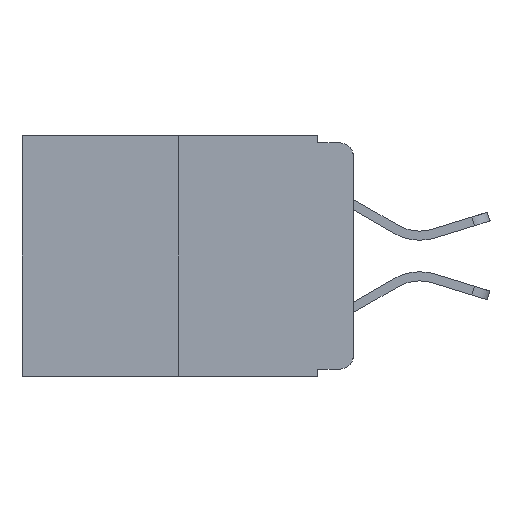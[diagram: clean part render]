
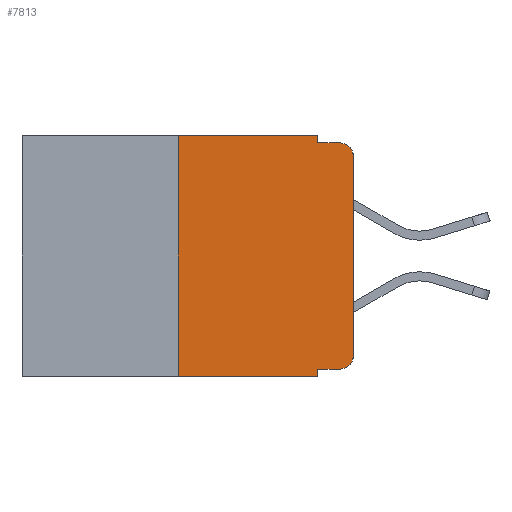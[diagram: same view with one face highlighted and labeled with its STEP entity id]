
A CAD part, left-side view. The second image highlights one B-rep face of the part: STEP entity #7813.
In plain terms, the highlighted planar face has unit normal (-1, 0, 0).
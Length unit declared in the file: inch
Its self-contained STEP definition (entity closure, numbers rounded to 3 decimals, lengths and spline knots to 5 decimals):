
#68 = AXIS2_PLACEMENT_3D ( 'NONE', #7513, #20662, #9401 ) ;
#79 = VECTOR ( 'NONE', #5910, 39.37008 ) ;
#618 = ORIENTED_EDGE ( 'NONE', *, *, #15214, .T. ) ;
#632 = DIRECTION ( 'NONE',  ( 0., -1., 0. ) ) ;
#761 = LINE ( 'NONE', #13624, #79 ) ;
#1089 = DIRECTION ( 'NONE',  ( 0., 0., -1. ) ) ;
#1434 = CIRCLE ( 'NONE', #7834, 0.02 ) ;
#1561 = EDGE_CURVE ( 'NONE', #3137, #16439, #16913, .T. ) ;
#1835 = LINE ( 'NONE', #22205, #12300 ) ;
#1865 = EDGE_CURVE ( 'NONE', #13426, #11484, #1434, .T. ) ;
#2576 = CARTESIAN_POINT ( 'NONE',  ( 0., 0.25, -0.343 ) ) ;
#2655 = CARTESIAN_POINT ( 'NONE',  ( 0., 0., 0. ) ) ;
#2921 = VECTOR ( 'NONE', #24233, 39.37008 ) ;
#3137 = VERTEX_POINT ( 'NONE', #23814 ) ;
#3278 = LINE ( 'NONE', #16063, #17871 ) ;
#3741 = ORIENTED_EDGE ( 'NONE', *, *, #1561, .T. ) ;
#3754 = AXIS2_PLACEMENT_3D ( 'NONE', #3768, #17104, #5752 ) ;
#3768 = CARTESIAN_POINT ( 'NONE',  ( 0., 0.473, 0. ) ) ;
#4059 = ORIENTED_EDGE ( 'NONE', *, *, #12887, .F. ) ;
#4904 = FACE_OUTER_BOUND ( 'NONE', #19486, .T. ) ;
#4918 = CARTESIAN_POINT ( 'NONE',  ( 0., 0.02, -0.01 ) ) ;
#5603 = ORIENTED_EDGE ( 'NONE', *, *, #19081, .T. ) ;
#5752 = DIRECTION ( 'NONE',  ( 0., 0., -1. ) ) ;
#5910 = DIRECTION ( 'NONE',  ( 0., 0., 1. ) ) ;
#6011 = VECTOR ( 'NONE', #632, 39.37008 ) ;
#6582 = DIRECTION ( 'NONE',  ( 0., 0., 1. ) ) ;
#6622 = LINE ( 'NONE', #14432, #6011 ) ;
#6765 = VERTEX_POINT ( 'NONE', #15989 ) ;
#7513 = CARTESIAN_POINT ( 'NONE',  ( 0., 0.02, -0.313 ) ) ;
#7595 = LINE ( 'NONE', #2655, #11539 ) ;
#7813 = ADVANCED_FACE ( 'NONE', ( #4904 ), #11496, .F. ) ;
#7834 = AXIS2_PLACEMENT_3D ( 'NONE', #23665, #23700, #21251 ) ;
#8142 = LINE ( 'NONE', #11283, #2921 ) ;
#9237 = VERTEX_POINT ( 'NONE', #12190 ) ;
#9401 = DIRECTION ( 'NONE',  ( 0., 0., -1. ) ) ;
#9455 = EDGE_CURVE ( 'NONE', #14515, #6765, #12429, .T. ) ;
#10920 = CARTESIAN_POINT ( 'NONE',  ( 0., 0.473, 0. ) ) ;
#11263 = CARTESIAN_POINT ( 'NONE',  ( 0., 0.02, -0.333 ) ) ;
#11283 = CARTESIAN_POINT ( 'NONE',  ( 0., 0.473, -0.343 ) ) ;
#11401 = VECTOR ( 'NONE', #16512, 39.37008 ) ;
#11484 = VERTEX_POINT ( 'NONE', #4918 ) ;
#11496 = PLANE ( 'NONE',  #3754 ) ;
#11539 = VECTOR ( 'NONE', #6582, 39.37008 ) ;
#11835 = VECTOR ( 'NONE', #12847, 39.37008 ) ;
#12190 = CARTESIAN_POINT ( 'NONE',  ( 0., 0., -0.313 ) ) ;
#12300 = VECTOR ( 'NONE', #1089, 39.37008 ) ;
#12429 = LINE ( 'NONE', #10920, #11835 ) ;
#12629 = VERTEX_POINT ( 'NONE', #14851 ) ;
#12847 = DIRECTION ( 'NONE',  ( 0., -1., 0. ) ) ;
#12887 = EDGE_CURVE ( 'NONE', #14483, #14515, #761, .T. ) ;
#13285 = CARTESIAN_POINT ( 'NONE',  ( 0., 0., -0.03 ) ) ;
#13357 = CARTESIAN_POINT ( 'NONE',  ( 0., 0.051, -0.333 ) ) ;
#13426 = VERTEX_POINT ( 'NONE', #13285 ) ;
#13624 = CARTESIAN_POINT ( 'NONE',  ( 0., 0.25, 0. ) ) ;
#13991 = EDGE_CURVE ( 'NONE', #3137, #16441, #1835, .T. ) ;
#14291 = CARTESIAN_POINT ( 'NONE',  ( 0., 0.25, 0. ) ) ;
#14432 = CARTESIAN_POINT ( 'NONE',  ( 0., 0.051, -0.01 ) ) ;
#14483 = VERTEX_POINT ( 'NONE', #2576 ) ;
#14515 = VERTEX_POINT ( 'NONE', #14291 ) ;
#14851 = CARTESIAN_POINT ( 'NONE',  ( 0., 0.051, -0.01 ) ) ;
#15214 = EDGE_CURVE ( 'NONE', #16439, #9237, #17437, .T. ) ;
#15421 = ORIENTED_EDGE ( 'NONE', *, *, #9455, .F. ) ;
#15921 = ORIENTED_EDGE ( 'NONE', *, *, #18143, .T. ) ;
#15989 = CARTESIAN_POINT ( 'NONE',  ( 0., 0.051, 0. ) ) ;
#16063 = CARTESIAN_POINT ( 'NONE',  ( 0., 0.051, 0. ) ) ;
#16439 = VERTEX_POINT ( 'NONE', #11263 ) ;
#16441 = VERTEX_POINT ( 'NONE', #18652 ) ;
#16512 = DIRECTION ( 'NONE',  ( 0., -1., 0. ) ) ;
#16588 = ORIENTED_EDGE ( 'NONE', *, *, #18829, .F. ) ;
#16913 = LINE ( 'NONE', #13357, #11401 ) ;
#17104 = DIRECTION ( 'NONE',  ( 1., 0., 0. ) ) ;
#17163 = ORIENTED_EDGE ( 'NONE', *, *, #13991, .F. ) ;
#17437 = CIRCLE ( 'NONE', #68, 0.02 ) ;
#17871 = VECTOR ( 'NONE', #21653, 39.37008 ) ;
#18143 = EDGE_CURVE ( 'NONE', #9237, #13426, #7595, .T. ) ;
#18652 = CARTESIAN_POINT ( 'NONE',  ( 0., 0.051, -0.343 ) ) ;
#18829 = EDGE_CURVE ( 'NONE', #6765, #12629, #3278, .T. ) ;
#18923 = ORIENTED_EDGE ( 'NONE', *, *, #1865, .T. ) ;
#19081 = EDGE_CURVE ( 'NONE', #14483, #16441, #8142, .T. ) ;
#19486 = EDGE_LOOP ( 'NONE', ( #15921, #18923, #21495, #16588, #15421, #4059, #5603, #17163, #3741, #618 ) ) ;
#20320 = EDGE_CURVE ( 'NONE', #12629, #11484, #6622, .T. ) ;
#20662 = DIRECTION ( 'NONE',  ( -1., 0., 0. ) ) ;
#21251 = DIRECTION ( 'NONE',  ( 0., 0., -1. ) ) ;
#21495 = ORIENTED_EDGE ( 'NONE', *, *, #20320, .F. ) ;
#21653 = DIRECTION ( 'NONE',  ( 0., 0., -1. ) ) ;
#22205 = CARTESIAN_POINT ( 'NONE',  ( 0., 0.051, 0. ) ) ;
#23665 = CARTESIAN_POINT ( 'NONE',  ( 0., 0.02, -0.03 ) ) ;
#23700 = DIRECTION ( 'NONE',  ( -1., 0., 0. ) ) ;
#23814 = CARTESIAN_POINT ( 'NONE',  ( 0., 0.051, -0.333 ) ) ;
#24233 = DIRECTION ( 'NONE',  ( 0., -1., 0. ) ) ;
